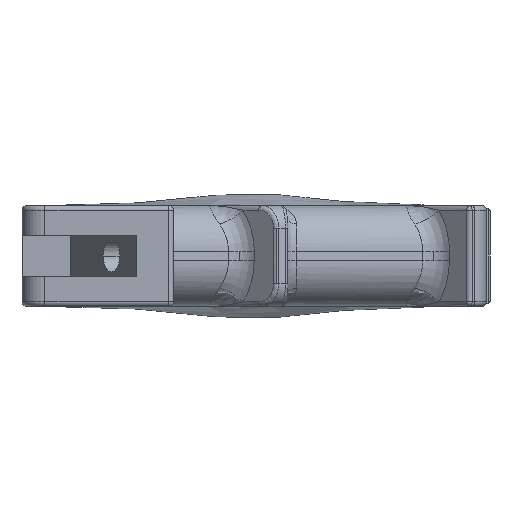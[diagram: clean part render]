
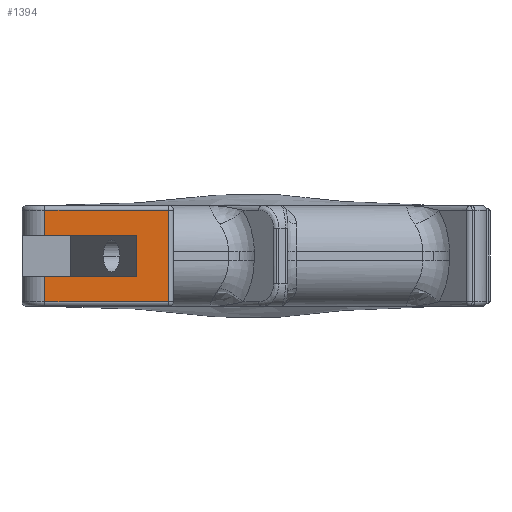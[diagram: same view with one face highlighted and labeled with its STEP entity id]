
A CAD part, left-side view. The second image highlights one B-rep face of the part: STEP entity #1394.
In plain terms, the highlighted planar face has unit normal (-1, 0, 0).
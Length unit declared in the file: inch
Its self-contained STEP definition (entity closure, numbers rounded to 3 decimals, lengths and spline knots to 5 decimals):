
#26 = VERTEX_POINT ( 'NONE', #4031 ) ;
#386 = PLANE ( 'NONE',  #1616 ) ;
#393 = VERTEX_POINT ( 'NONE', #747 ) ;
#503 = ORIENTED_EDGE ( 'NONE', *, *, #633, .F. ) ;
#598 = EDGE_CURVE ( 'NONE', #26, #8191, #3434, .T. ) ;
#633 = EDGE_CURVE ( 'NONE', #5917, #393, #5269, .T. ) ;
#634 = LINE ( 'NONE', #1262, #7684 ) ;
#693 = EDGE_CURVE ( 'NONE', #8191, #5917, #8614, .T. ) ;
#707 = EDGE_CURVE ( 'NONE', #8002, #26, #8172, .T. ) ;
#721 = EDGE_CURVE ( 'NONE', #8200, #5515, #6207, .T. ) ;
#747 = CARTESIAN_POINT ( 'NONE',  ( 0., 1.10236, -0.3937 ) ) ;
#872 = ORIENTED_EDGE ( 'NONE', *, *, #598, .F. ) ;
#888 = CARTESIAN_POINT ( 'NONE',  ( 0., 0.03937, 0.3937 ) ) ;
#1095 = ORIENTED_EDGE ( 'NONE', *, *, #4728, .F. ) ;
#1115 = CARTESIAN_POINT ( 'NONE',  ( 0., 0.03937, -0.3937 ) ) ;
#1160 = DIRECTION ( 'NONE',  ( 0., 0., 1. ) ) ;
#1170 = DIRECTION ( 'NONE',  ( 0., 1., 0. ) ) ;
#1177 = VECTOR ( 'NONE', #1567, 39.37008 ) ;
#1207 = CARTESIAN_POINT ( 'NONE',  ( 0., 0.03937, -0.3937 ) ) ;
#1262 = CARTESIAN_POINT ( 'NONE',  ( 0., 1.10236, -0.3937 ) ) ;
#1263 = LINE ( 'NONE', #3182, #4682 ) ;
#1394 = ADVANCED_FACE ( 'NONE', ( #7117 ), #386, .T. ) ;
#1453 = DIRECTION ( 'NONE',  ( 0., -1., 0. ) ) ;
#1480 = CARTESIAN_POINT ( 'NONE',  ( 0., 1.10236, 0.3937 ) ) ;
#1567 = DIRECTION ( 'NONE',  ( 0., 0., 1. ) ) ;
#1616 = AXIS2_PLACEMENT_3D ( 'NONE', #1115, #1840, #6579 ) ;
#1627 = CARTESIAN_POINT ( 'NONE',  ( 0., 0.31496, -0.17717 ) ) ;
#1631 = VECTOR ( 'NONE', #1170, 39.37008 ) ;
#1663 = DIRECTION ( 'NONE',  ( 0., 0., -1. ) ) ;
#1818 = CARTESIAN_POINT ( 'NONE',  ( 0., 1.10236, 0.17717 ) ) ;
#1840 = DIRECTION ( 'NONE',  ( -1., 0., 0. ) ) ;
#1855 = CARTESIAN_POINT ( 'NONE',  ( 0., 0.03937, 0.3937 ) ) ;
#1950 = DIRECTION ( 'NONE',  ( 0., -1., 0. ) ) ;
#2313 = VERTEX_POINT ( 'NONE', #3084 ) ;
#2325 = ORIENTED_EDGE ( 'NONE', *, *, #4869, .F. ) ;
#2492 = DIRECTION ( 'NONE',  ( 0., 1., 0. ) ) ;
#2549 = ORIENTED_EDGE ( 'NONE', *, *, #4929, .F. ) ;
#2603 = VECTOR ( 'NONE', #1160, 39.37008 ) ;
#3084 = CARTESIAN_POINT ( 'NONE',  ( 0., 1.10236, -0.17717 ) ) ;
#3182 = CARTESIAN_POINT ( 'NONE',  ( 0., 0.31496, 0.17717 ) ) ;
#3434 = LINE ( 'NONE', #1480, #7020 ) ;
#3677 = EDGE_LOOP ( 'NONE', ( #2325, #2549, #503, #6151, #872, #6358, #1095, #8117 ) ) ;
#3717 = CARTESIAN_POINT ( 'NONE',  ( 0., 0.03937, -0.3937 ) ) ;
#4031 = CARTESIAN_POINT ( 'NONE',  ( 0., 1.10236, 0.3937 ) ) ;
#4600 = VECTOR ( 'NONE', #1663, 39.37008 ) ;
#4682 = VECTOR ( 'NONE', #2492, 39.37008 ) ;
#4728 = EDGE_CURVE ( 'NONE', #5515, #8002, #1263, .T. ) ;
#4869 = EDGE_CURVE ( 'NONE', #2313, #8200, #5879, .T. ) ;
#4929 = EDGE_CURVE ( 'NONE', #393, #2313, #634, .T. ) ;
#5269 = LINE ( 'NONE', #1207, #1631 ) ;
#5349 = CARTESIAN_POINT ( 'NONE',  ( 0., 0.31496, 0.17717 ) ) ;
#5384 = DIRECTION ( 'NONE',  ( 0., 0., 1. ) ) ;
#5515 = VERTEX_POINT ( 'NONE', #5349 ) ;
#5714 = CARTESIAN_POINT ( 'NONE',  ( 0., 0.31496, -0.17717 ) ) ;
#5879 = LINE ( 'NONE', #6031, #7844 ) ;
#5917 = VERTEX_POINT ( 'NONE', #3717 ) ;
#6031 = CARTESIAN_POINT ( 'NONE',  ( 0., 1.10236, -0.17717 ) ) ;
#6151 = ORIENTED_EDGE ( 'NONE', *, *, #693, .F. ) ;
#6207 = LINE ( 'NONE', #1627, #2603 ) ;
#6358 = ORIENTED_EDGE ( 'NONE', *, *, #707, .F. ) ;
#6579 = DIRECTION ( 'NONE',  ( 0., 0., 1. ) ) ;
#7020 = VECTOR ( 'NONE', #1453, 39.37008 ) ;
#7117 = FACE_OUTER_BOUND ( 'NONE', #3677, .T. ) ;
#7672 = CARTESIAN_POINT ( 'NONE',  ( 0., 1.10236, 0.17717 ) ) ;
#7684 = VECTOR ( 'NONE', #5384, 39.37008 ) ;
#7844 = VECTOR ( 'NONE', #1950, 39.37008 ) ;
#8002 = VERTEX_POINT ( 'NONE', #7672 ) ;
#8117 = ORIENTED_EDGE ( 'NONE', *, *, #721, .F. ) ;
#8172 = LINE ( 'NONE', #1818, #1177 ) ;
#8191 = VERTEX_POINT ( 'NONE', #888 ) ;
#8200 = VERTEX_POINT ( 'NONE', #5714 ) ;
#8614 = LINE ( 'NONE', #1855, #4600 ) ;
